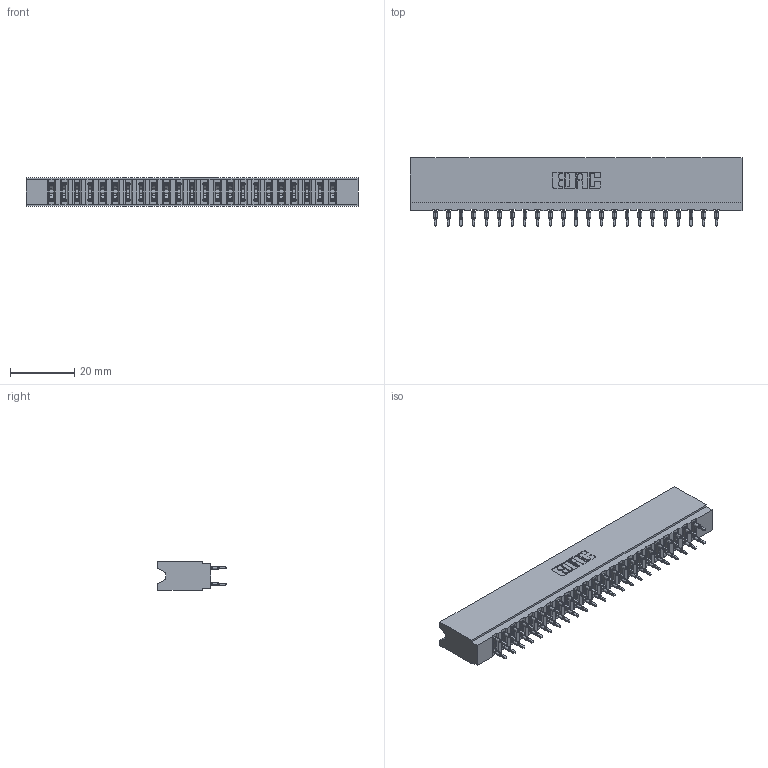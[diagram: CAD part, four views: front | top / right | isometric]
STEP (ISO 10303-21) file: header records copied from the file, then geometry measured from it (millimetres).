
FILE_DESCRIPTION (( 'STEP AP203' ), '1' );
FILE_NAME ('737-046-525-206.STEP', '2020-09-11T04:07:25', ( '' ), ( '' ), 'SwSTEP 2.0', 'SolidWorks 2020', '' );
FILE_SCHEMA (( 'CONFIG_CONTROL_DESIGN' ));
Length unit declared in the file: inch
Products named in the file (3): 737-046-525-206; 745-292-001_525; 737 Part_Insulator Option - 06
Assembly tree (47 placements, depth 2):
  737-046-525-206
    737 Part_Insulator Option - 06
    745-292-001_525  x46
Bounding box: 102.97 x 21.22 x 8.89 mm (x, y, z)
Volume: 10265.6 mm3; surface area: 14449.9 mm2
Topology: 47 solids, 47 shells, 4235 faces, 11389 edges, 7162 vertices
Faces by surface type: plane 2194, bspline 920, cylinder 845, torus 276
Entity records: 42067 total; most frequent: CARTESIAN_POINT 7810, ORIENTED_EDGE 7208, DIRECTION 6308, EDGE_CURVE 3604, VECTOR 3284, LINE 3284, VERTEX_POINT 2302, AXIS2_PLACEMENT_3D 1512
